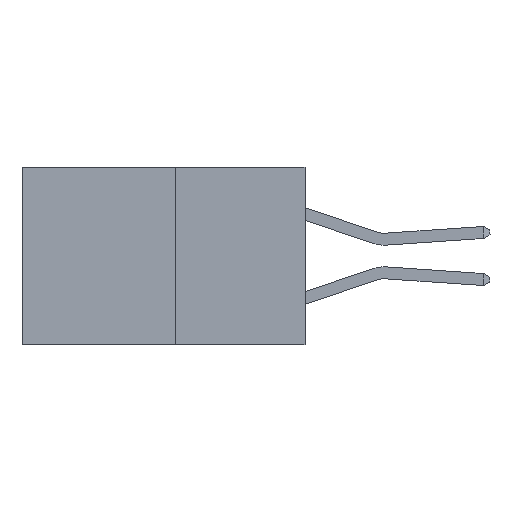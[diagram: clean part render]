
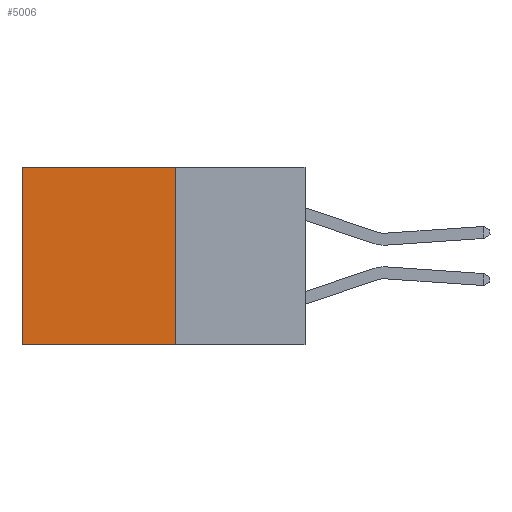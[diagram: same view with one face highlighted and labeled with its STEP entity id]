
A CAD part, left-side view. The second image highlights one B-rep face of the part: STEP entity #5006.
In plain terms, the highlighted planar face has unit normal (-1, 0, 0).
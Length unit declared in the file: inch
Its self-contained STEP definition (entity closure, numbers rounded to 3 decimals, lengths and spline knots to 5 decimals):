
#229 = LINE ( 'NONE', #8434, #9044 ) ;
#1887 = EDGE_CURVE ( 'NONE', #10150, #8745, #2363, .T. ) ;
#2363 = LINE ( 'NONE', #10773, #10900 ) ;
#2367 = DIRECTION ( 'NONE',  ( 0., 1., 0. ) ) ;
#2465 = EDGE_LOOP ( 'NONE', ( #9360, #3318, #8430, #2928 ) ) ;
#2836 = CARTESIAN_POINT ( 'NONE',  ( 0.277, 0.27, -0.37 ) ) ;
#2928 = ORIENTED_EDGE ( 'NONE', *, *, #1887, .T. ) ;
#2954 = CARTESIAN_POINT ( 'NONE',  ( 0.277, 0.59, -0.37 ) ) ;
#3005 = EDGE_CURVE ( 'NONE', #8745, #8667, #6382, .T. ) ;
#3318 = ORIENTED_EDGE ( 'NONE', *, *, #4308, .F. ) ;
#4223 = VERTEX_POINT ( 'NONE', #2836 ) ;
#4308 = EDGE_CURVE ( 'NONE', #4223, #8667, #8975, .T. ) ;
#5006 = ADVANCED_FACE ( 'NONE', ( #6345 ), #6178, .F. ) ;
#6178 = PLANE ( 'NONE',  #10203 ) ;
#6270 = DIRECTION ( 'NONE',  ( 0., 0., -1. ) ) ;
#6345 = FACE_OUTER_BOUND ( 'NONE', #2465, .T. ) ;
#6382 = LINE ( 'NONE', #2954, #10455 ) ;
#6616 = VECTOR ( 'NONE', #2367, 39.37008 ) ;
#7105 = DIRECTION ( 'NONE',  ( 1., 0., 0. ) ) ;
#7635 = EDGE_CURVE ( 'NONE', #10150, #4223, #229, .T. ) ;
#7715 = CARTESIAN_POINT ( 'NONE',  ( 0.277, 0.27, 0. ) ) ;
#8430 = ORIENTED_EDGE ( 'NONE', *, *, #7635, .F. ) ;
#8434 = CARTESIAN_POINT ( 'NONE',  ( 0.277, 0.27, -0.37 ) ) ;
#8536 = DIRECTION ( 'NONE',  ( 0., 0., -1. ) ) ;
#8612 = CARTESIAN_POINT ( 'NONE',  ( 0.277, 0.27, -0.37 ) ) ;
#8667 = VERTEX_POINT ( 'NONE', #9918 ) ;
#8745 = VERTEX_POINT ( 'NONE', #9177 ) ;
#8975 = LINE ( 'NONE', #10751, #6616 ) ;
#9044 = VECTOR ( 'NONE', #8536, 39.37008 ) ;
#9177 = CARTESIAN_POINT ( 'NONE',  ( 0.277, 0.59, 0. ) ) ;
#9360 = ORIENTED_EDGE ( 'NONE', *, *, #3005, .T. ) ;
#9918 = CARTESIAN_POINT ( 'NONE',  ( 0.277, 0.59, -0.37 ) ) ;
#10150 = VERTEX_POINT ( 'NONE', #7715 ) ;
#10203 = AXIS2_PLACEMENT_3D ( 'NONE', #8612, #7105, #10977 ) ;
#10455 = VECTOR ( 'NONE', #6270, 39.37008 ) ;
#10619 = DIRECTION ( 'NONE',  ( 0., 1., 0. ) ) ;
#10751 = CARTESIAN_POINT ( 'NONE',  ( 0.277, 0.27, -0.37 ) ) ;
#10773 = CARTESIAN_POINT ( 'NONE',  ( 0.277, 0.27, 0. ) ) ;
#10900 = VECTOR ( 'NONE', #10619, 39.37008 ) ;
#10977 = DIRECTION ( 'NONE',  ( 0., 0., -1. ) ) ;
